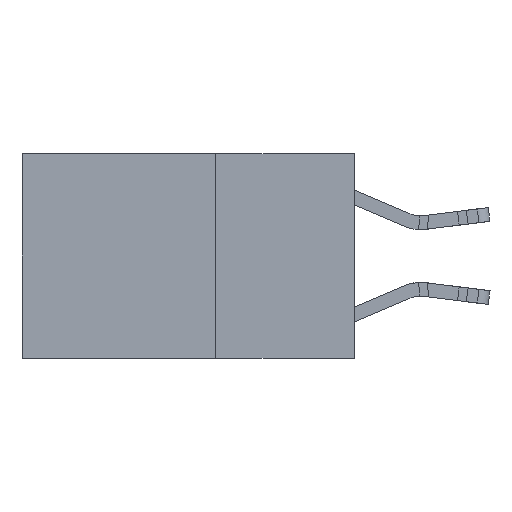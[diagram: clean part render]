
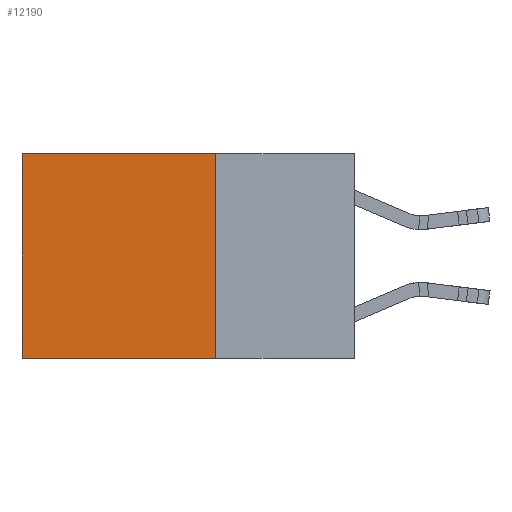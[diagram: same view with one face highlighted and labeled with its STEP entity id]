
A CAD part, left-side view. The second image highlights one B-rep face of the part: STEP entity #12190.
In plain terms, the highlighted planar face has unit normal (-1, 0, 0).
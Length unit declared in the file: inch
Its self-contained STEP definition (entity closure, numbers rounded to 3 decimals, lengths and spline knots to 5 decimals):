
#2356 = EDGE_LOOP ( 'NONE', ( #21059, #17628, #18694, #27183 ) ) ;
#2663 = AXIS2_PLACEMENT_3D ( 'NONE', #20235, #27246, #6442 ) ;
#4003 = VECTOR ( 'NONE', #23327, 39.37008 ) ;
#4095 = CARTESIAN_POINT ( 'NONE',  ( 0.2625, 0.25, -0.37 ) ) ;
#4455 = EDGE_CURVE ( 'NONE', #15826, #12578, #6100, .T. ) ;
#4459 = CARTESIAN_POINT ( 'NONE',  ( 0.2625, 0.25, -0.37 ) ) ;
#5730 = VECTOR ( 'NONE', #29770, 39.37008 ) ;
#5839 = CARTESIAN_POINT ( 'NONE',  ( 0.2625, 0.6, -0.37 ) ) ;
#6100 = LINE ( 'NONE', #10938, #17929 ) ;
#6442 = DIRECTION ( 'NONE',  ( 0., 0., -1. ) ) ;
#6705 = CARTESIAN_POINT ( 'NONE',  ( 0.2625, 0.6, 0. ) ) ;
#7595 = EDGE_CURVE ( 'NONE', #15826, #13468, #27887, .T. ) ;
#9002 = LINE ( 'NONE', #27387, #29703 ) ;
#10938 = CARTESIAN_POINT ( 'NONE',  ( 0.2625, 0.25, 0. ) ) ;
#12190 = ADVANCED_FACE ( 'NONE', ( #18095 ), #27393, .F. ) ;
#12578 = VERTEX_POINT ( 'NONE', #6705 ) ;
#13468 = VERTEX_POINT ( 'NONE', #4459 ) ;
#15826 = VERTEX_POINT ( 'NONE', #26984 ) ;
#15840 = DIRECTION ( 'NONE',  ( 0., 0., -1. ) ) ;
#17628 = ORIENTED_EDGE ( 'NONE', *, *, #27314, .F. ) ;
#17929 = VECTOR ( 'NONE', #24466, 39.37008 ) ;
#18095 = FACE_OUTER_BOUND ( 'NONE', #2356, .T. ) ;
#18694 = ORIENTED_EDGE ( 'NONE', *, *, #7595, .F. ) ;
#19309 = EDGE_CURVE ( 'NONE', #12578, #20361, #9002, .T. ) ;
#20235 = CARTESIAN_POINT ( 'NONE',  ( 0.2625, 0.25, 0. ) ) ;
#20361 = VERTEX_POINT ( 'NONE', #5839 ) ;
#21059 = ORIENTED_EDGE ( 'NONE', *, *, #19309, .T. ) ;
#23327 = DIRECTION ( 'NONE',  ( 0., 0., -1. ) ) ;
#24466 = DIRECTION ( 'NONE',  ( 0., 1., 0. ) ) ;
#25893 = CARTESIAN_POINT ( 'NONE',  ( 0.2625, 0.25, 0. ) ) ;
#26984 = CARTESIAN_POINT ( 'NONE',  ( 0.2625, 0.25, 0. ) ) ;
#27183 = ORIENTED_EDGE ( 'NONE', *, *, #4455, .T. ) ;
#27199 = LINE ( 'NONE', #4095, #5730 ) ;
#27246 = DIRECTION ( 'NONE',  ( 1., 0., 0. ) ) ;
#27314 = EDGE_CURVE ( 'NONE', #13468, #20361, #27199, .T. ) ;
#27387 = CARTESIAN_POINT ( 'NONE',  ( 0.2625, 0.6, 0. ) ) ;
#27393 = PLANE ( 'NONE',  #2663 ) ;
#27887 = LINE ( 'NONE', #25893, #4003 ) ;
#29703 = VECTOR ( 'NONE', #15840, 39.37008 ) ;
#29770 = DIRECTION ( 'NONE',  ( 0., 1., 0. ) ) ;
